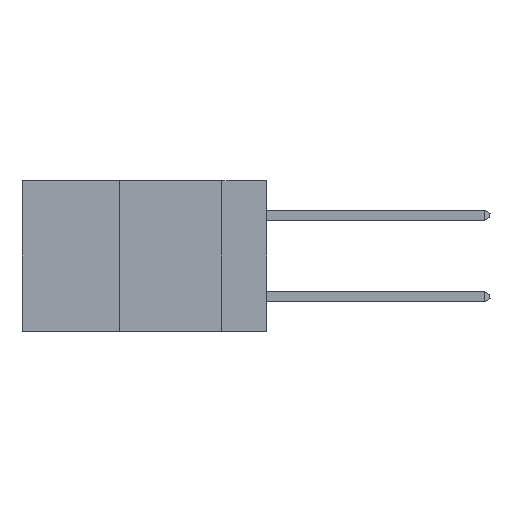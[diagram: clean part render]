
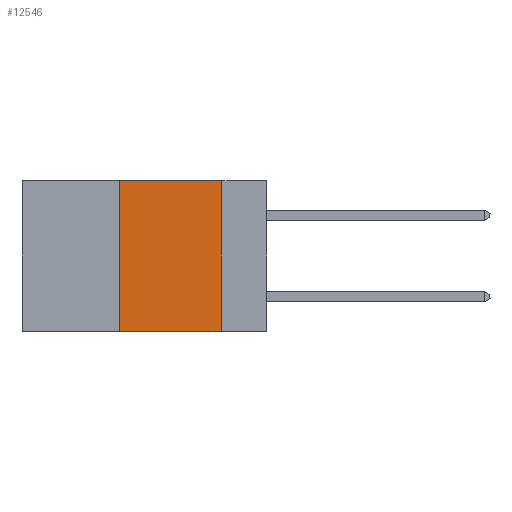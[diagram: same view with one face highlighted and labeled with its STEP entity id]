
A CAD part, left-side view. The second image highlights one B-rep face of the part: STEP entity #12546.
In plain terms, the highlighted planar face has unit normal (-1, 0, 0).
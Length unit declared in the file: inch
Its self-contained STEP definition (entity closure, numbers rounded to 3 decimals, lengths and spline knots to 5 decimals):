
#7252 = DIRECTION ( 'NONE',  ( 0., 0., -1. ) ) ;
#7532 = VERTEX_POINT ( 'NONE', #11463 ) ;
#8095 = VECTOR ( 'NONE', #7252, 39.37008 ) ;
#8222 = VECTOR ( 'NONE', #28068, 39.37008 ) ;
#8244 = VERTEX_POINT ( 'NONE', #31925 ) ;
#8329 = FACE_OUTER_BOUND ( 'NONE', #31458, .T. ) ;
#8566 = VECTOR ( 'NONE', #18920, 39.37008 ) ;
#10103 = AXIS2_PLACEMENT_3D ( 'NONE', #11713, #29460, #14244 ) ;
#11050 = CARTESIAN_POINT ( 'NONE',  ( 0., 0.36, -0.37 ) ) ;
#11463 = CARTESIAN_POINT ( 'NONE',  ( 0., 0.11, -0.37 ) ) ;
#11713 = CARTESIAN_POINT ( 'NONE',  ( 0., 0.6, 0. ) ) ;
#12296 = CARTESIAN_POINT ( 'NONE',  ( 0., 0.11, 0. ) ) ;
#12458 = CARTESIAN_POINT ( 'NONE',  ( 0., 0.6, -0.37 ) ) ;
#12546 = ADVANCED_FACE ( 'NONE', ( #8329 ), #21860, .F. ) ;
#12595 = VERTEX_POINT ( 'NONE', #27196 ) ;
#12819 = CARTESIAN_POINT ( 'NONE',  ( 0., 0.6, 0. ) ) ;
#12849 = ORIENTED_EDGE ( 'NONE', *, *, #15067, .F. ) ;
#13238 = EDGE_CURVE ( 'NONE', #12595, #8244, #15010, .T. ) ;
#13848 = CARTESIAN_POINT ( 'NONE',  ( 0., 0.36, 0. ) ) ;
#14066 = LINE ( 'NONE', #12296, #8095 ) ;
#14079 = VECTOR ( 'NONE', #30220, 39.37008 ) ;
#14244 = DIRECTION ( 'NONE',  ( 0., 0., -1. ) ) ;
#14452 = ORIENTED_EDGE ( 'NONE', *, *, #32834, .T. ) ;
#15010 = LINE ( 'NONE', #12819, #8222 ) ;
#15067 = EDGE_CURVE ( 'NONE', #8244, #7532, #14066, .T. ) ;
#15395 = VERTEX_POINT ( 'NONE', #11050 ) ;
#18920 = DIRECTION ( 'NONE',  ( 0., 0., 1. ) ) ;
#21860 = PLANE ( 'NONE',  #10103 ) ;
#22366 = EDGE_CURVE ( 'NONE', #15395, #12595, #28859, .T. ) ;
#26424 = ORIENTED_EDGE ( 'NONE', *, *, #13238, .F. ) ;
#27196 = CARTESIAN_POINT ( 'NONE',  ( 0., 0.36, 0. ) ) ;
#27228 = ORIENTED_EDGE ( 'NONE', *, *, #22366, .F. ) ;
#27652 = LINE ( 'NONE', #12458, #14079 ) ;
#28068 = DIRECTION ( 'NONE',  ( 0., -1., 0. ) ) ;
#28859 = LINE ( 'NONE', #13848, #8566 ) ;
#29460 = DIRECTION ( 'NONE',  ( 1., 0., 0. ) ) ;
#30220 = DIRECTION ( 'NONE',  ( 0., -1., 0. ) ) ;
#31458 = EDGE_LOOP ( 'NONE', ( #12849, #26424, #27228, #14452 ) ) ;
#31925 = CARTESIAN_POINT ( 'NONE',  ( 0., 0.11, 0. ) ) ;
#32834 = EDGE_CURVE ( 'NONE', #15395, #7532, #27652, .T. ) ;
